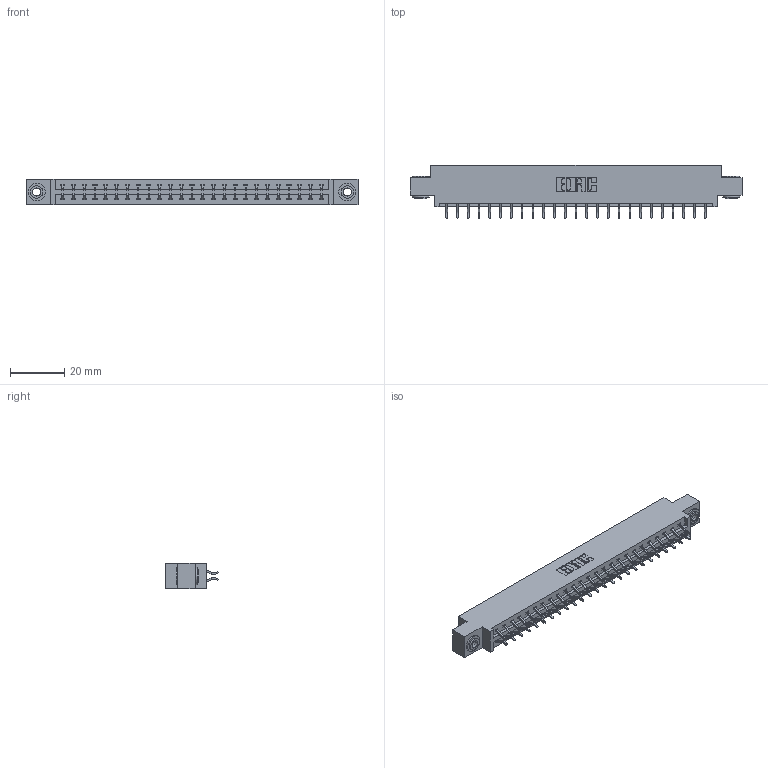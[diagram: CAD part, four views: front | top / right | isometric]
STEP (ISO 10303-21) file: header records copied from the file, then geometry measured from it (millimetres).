
FILE_DESCRIPTION (( 'STEP AP203' ), '1' );
FILE_NAME ('387-050-556-803.STEP', '2018-09-20T08:57:22', ( '' ), ( '' ), 'SwSTEP 2.0', 'SolidWorks 2016', '' );
FILE_SCHEMA (( 'CONFIG_CONTROL_DESIGN' ));
Length unit declared in the file: inch
Products named in the file (4): 337 Part_0.170 Offset - 0.156 Dia-TH; 345-292-001_556 Tail; 345-250-002_345-250-002-102; 387-050-556-803
Assembly tree (53 placements, depth 2):
  387-050-556-803
    337 Part_0.170 Offset - 0.156 Dia-TH
    345-292-001_556 Tail  x50
    345-250-002_345-250-002-102  x2
Bounding box: 122.07 x 19.57 x 9.4 mm (x, y, z)
Volume: 12538.6 mm3; surface area: 14289.2 mm2
Topology: 53 solids, 53 shells, 3156 faces, 9349 edges, 6162 vertices
Faces by surface type: plane 2184, cylinder 964, cone 8
Entity records: 22584 total; most frequent: CARTESIAN_POINT 3809, ORIENTED_EDGE 3726, DIRECTION 3293, EDGE_CURVE 1863, VECTOR 1703, LINE 1703, VERTEX_POINT 1238, AXIS2_PLACEMENT_3D 795
